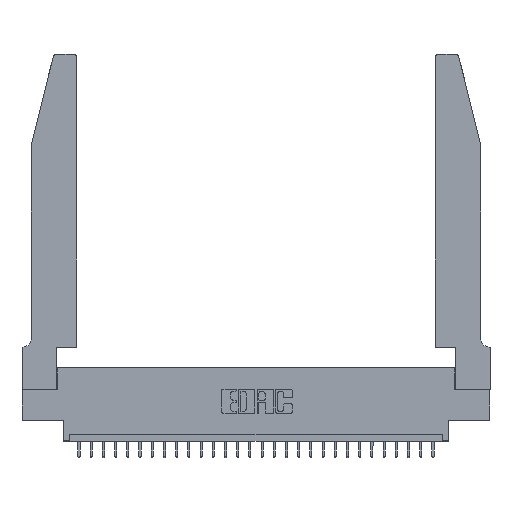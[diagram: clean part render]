
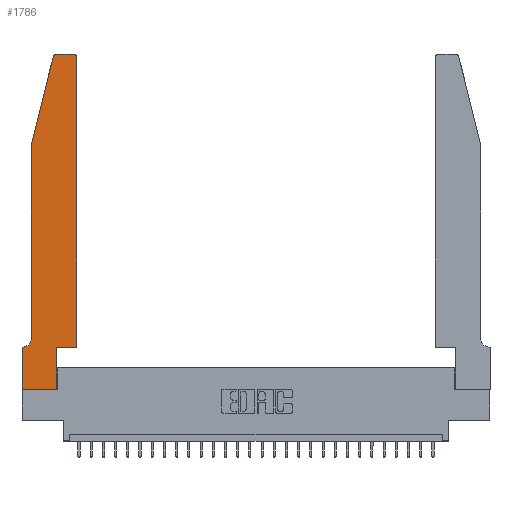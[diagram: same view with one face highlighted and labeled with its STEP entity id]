
A CAD part, top view. The second image highlights one B-rep face of the part: STEP entity #1786.
In plain terms, the highlighted planar face has unit normal (0, 0, 1).
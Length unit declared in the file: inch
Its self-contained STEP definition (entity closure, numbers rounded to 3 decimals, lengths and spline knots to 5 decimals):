
#113 = VERTEX_POINT ( 'NONE', #26144 ) ;
#346 = ORIENTED_EDGE ( 'NONE', *, *, #4771, .T. ) ;
#759 = LINE ( 'NONE', #21022, #28540 ) ;
#939 = CARTESIAN_POINT ( 'NONE',  ( 0., 0., 0.37 ) ) ;
#1081 = VECTOR ( 'NONE', #6159, 39.37008 ) ;
#1107 = EDGE_CURVE ( 'NONE', #24085, #16283, #13024, .T. ) ;
#1116 = EDGE_CURVE ( 'NONE', #14384, #13905, #27344, .T. ) ;
#1422 = CARTESIAN_POINT ( 'NONE',  ( 0.0755, 2., 0.37 ) ) ;
#1423 = LINE ( 'NONE', #18894, #9993 ) ;
#1582 = CARTESIAN_POINT ( 'NONE',  ( 0.0755, 2., 0.37 ) ) ;
#1786 = ADVANCED_FACE ( 'NONE', ( #25064 ), #11486, .T. ) ;
#2566 = CARTESIAN_POINT ( 'NONE',  ( 0.0055, 0.42, 0.37 ) ) ;
#2637 = EDGE_CURVE ( 'NONE', #11356, #17026, #1423, .T. ) ;
#3624 = DIRECTION ( 'NONE',  ( 0., 1., 0. ) ) ;
#3941 = CARTESIAN_POINT ( 'NONE',  ( 0.0055, 0.35, 0.37 ) ) ;
#4277 = DIRECTION ( 'NONE',  ( 0., -1., 0. ) ) ;
#4666 = VECTOR ( 'NONE', #4277, 39.37008 ) ;
#4771 = EDGE_CURVE ( 'NONE', #113, #11356, #10978, .T. ) ;
#5021 = CARTESIAN_POINT ( 'NONE',  ( 0.2865, 0.35, 0.37 ) ) ;
#5240 = VERTEX_POINT ( 'NONE', #14966 ) ;
#5389 = ORIENTED_EDGE ( 'NONE', *, *, #12467, .T. ) ;
#5430 = LINE ( 'NONE', #18927, #10160 ) ;
#5456 = DIRECTION ( 'NONE',  ( 0., 1., 0. ) ) ;
#5541 = CIRCLE ( 'NONE', #9285, 0.03 ) ;
#5639 = CARTESIAN_POINT ( 'NONE',  ( 0.284, 2.75, 0.37 ) ) ;
#6159 = DIRECTION ( 'NONE',  ( 0., -1., 0. ) ) ;
#6169 = ORIENTED_EDGE ( 'NONE', *, *, #23063, .T. ) ;
#6277 = ORIENTED_EDGE ( 'NONE', *, *, #1107, .T. ) ;
#6427 = VECTOR ( 'NONE', #3624, 39.37008 ) ;
#6808 = DIRECTION ( 'NONE',  ( 1., 0., 0. ) ) ;
#7432 = ORIENTED_EDGE ( 'NONE', *, *, #21163, .T. ) ;
#7960 = EDGE_CURVE ( 'NONE', #27214, #5240, #5430, .T. ) ;
#8190 = DIRECTION ( 'NONE',  ( 1., 0., 0. ) ) ;
#8300 = EDGE_CURVE ( 'NONE', #28111, #24085, #5541, .T. ) ;
#8770 = DIRECTION ( 'NONE',  ( -0.239, -0.971, 0. ) ) ;
#9285 = AXIS2_PLACEMENT_3D ( 'NONE', #19889, #18239, #6808 ) ;
#9444 = AXIS2_PLACEMENT_3D ( 'NONE', #2566, #28035, #25078 ) ;
#9508 = CARTESIAN_POINT ( 'NONE',  ( 0.4205, 2.75, 0.37 ) ) ;
#9993 = VECTOR ( 'NONE', #27955, 39.37008 ) ;
#10160 = VECTOR ( 'NONE', #8190, 39.37008 ) ;
#10300 = ORIENTED_EDGE ( 'NONE', *, *, #7960, .T. ) ;
#10596 = EDGE_CURVE ( 'NONE', #10987, #25394, #17300, .T. ) ;
#10978 = LINE ( 'NONE', #21729, #1081 ) ;
#10987 = VERTEX_POINT ( 'NONE', #25023 ) ;
#11010 = EDGE_CURVE ( 'NONE', #16283, #14384, #15411, .T. ) ;
#11028 = CARTESIAN_POINT ( 'NONE',  ( 0.25487, 2.72718, 0.37 ) ) ;
#11356 = VERTEX_POINT ( 'NONE', #939 ) ;
#11486 = PLANE ( 'NONE',  #28354 ) ;
#12087 = DIRECTION ( 'NONE',  ( -1., 0., 0. ) ) ;
#12219 = ORIENTED_EDGE ( 'NONE', *, *, #10596, .T. ) ;
#12467 = EDGE_CURVE ( 'NONE', #5240, #10987, #15061, .T. ) ;
#13024 = LINE ( 'NONE', #1582, #20252 ) ;
#13569 = AXIS2_PLACEMENT_3D ( 'NONE', #17232, #15301, #26095 ) ;
#13905 = VERTEX_POINT ( 'NONE', #3941 ) ;
#14140 = CARTESIAN_POINT ( 'NONE',  ( 0., 0.35, 0.37 ) ) ;
#14181 = LINE ( 'NONE', #18862, #22955 ) ;
#14384 = VERTEX_POINT ( 'NONE', #16089 ) ;
#14966 = CARTESIAN_POINT ( 'NONE',  ( 0.4505, 0.35, 0.37 ) ) ;
#15061 = LINE ( 'NONE', #28258, #6427 ) ;
#15301 = DIRECTION ( 'NONE',  ( 0., 0., 1. ) ) ;
#15411 = LINE ( 'NONE', #24442, #4666 ) ;
#16089 = CARTESIAN_POINT ( 'NONE',  ( 0.0755, 0.42, 0.37 ) ) ;
#16283 = VERTEX_POINT ( 'NONE', #1422 ) ;
#16498 = DIRECTION ( 'NONE',  ( 1., 0., 0. ) ) ;
#17026 = VERTEX_POINT ( 'NONE', #25400 ) ;
#17232 = CARTESIAN_POINT ( 'NONE',  ( 0.4205, 2.72, 0.37 ) ) ;
#17300 = CIRCLE ( 'NONE', #13569, 0.03 ) ;
#18239 = DIRECTION ( 'NONE',  ( 0., 0., 1. ) ) ;
#18862 = CARTESIAN_POINT ( 'NONE',  ( 0.2605, 2.75, 0.37 ) ) ;
#18894 = CARTESIAN_POINT ( 'NONE',  ( 0., 0., 0.37 ) ) ;
#18927 = CARTESIAN_POINT ( 'NONE',  ( 0.4505, 0.35, 0.37 ) ) ;
#18991 = CARTESIAN_POINT ( 'NONE',  ( 0.0755, 0.35, 0.37 ) ) ;
#19889 = CARTESIAN_POINT ( 'NONE',  ( 0.284, 2.72, 0.37 ) ) ;
#20252 = VECTOR ( 'NONE', #8770, 39.37008 ) ;
#20440 = ORIENTED_EDGE ( 'NONE', *, *, #1116, .T. ) ;
#21022 = CARTESIAN_POINT ( 'NONE',  ( 0.2865, 0.35, 0.37 ) ) ;
#21163 = EDGE_CURVE ( 'NONE', #25394, #28111, #14181, .T. ) ;
#21257 = ORIENTED_EDGE ( 'NONE', *, *, #11010, .T. ) ;
#21729 = CARTESIAN_POINT ( 'NONE',  ( 0., 0., 0.37 ) ) ;
#22814 = VECTOR ( 'NONE', #12087, 39.37008 ) ;
#22955 = VECTOR ( 'NONE', #25975, 39.37008 ) ;
#23063 = EDGE_CURVE ( 'NONE', #13905, #113, #23875, .T. ) ;
#23726 = EDGE_CURVE ( 'NONE', #17026, #27214, #759, .T. ) ;
#23875 = LINE ( 'NONE', #18991, #22814 ) ;
#24085 = VERTEX_POINT ( 'NONE', #11028 ) ;
#24242 = EDGE_LOOP ( 'NONE', ( #7432, #28319, #6277, #21257, #20440, #6169, #346, #29160, #25777, #10300, #5389, #12219 ) ) ;
#24442 = CARTESIAN_POINT ( 'NONE',  ( 0.0755, 2., 0.37 ) ) ;
#25023 = CARTESIAN_POINT ( 'NONE',  ( 0.4505, 2.72, 0.37 ) ) ;
#25064 = FACE_OUTER_BOUND ( 'NONE', #24242, .T. ) ;
#25078 = DIRECTION ( 'NONE',  ( -1., 0., 0. ) ) ;
#25341 = DIRECTION ( 'NONE',  ( 0., 0., 1. ) ) ;
#25394 = VERTEX_POINT ( 'NONE', #9508 ) ;
#25400 = CARTESIAN_POINT ( 'NONE',  ( 0.2865, 0., 0.37 ) ) ;
#25777 = ORIENTED_EDGE ( 'NONE', *, *, #23726, .T. ) ;
#25975 = DIRECTION ( 'NONE',  ( -1., 0., 0. ) ) ;
#26095 = DIRECTION ( 'NONE',  ( 1., 0., 0. ) ) ;
#26144 = CARTESIAN_POINT ( 'NONE',  ( 0., 0.35, 0.37 ) ) ;
#27214 = VERTEX_POINT ( 'NONE', #5021 ) ;
#27344 = CIRCLE ( 'NONE', #9444, 0.07 ) ;
#27955 = DIRECTION ( 'NONE',  ( 1., 0., 0. ) ) ;
#28035 = DIRECTION ( 'NONE',  ( 0., 0., -1. ) ) ;
#28111 = VERTEX_POINT ( 'NONE', #5639 ) ;
#28258 = CARTESIAN_POINT ( 'NONE',  ( 0.4505, 0.35, 0.37 ) ) ;
#28319 = ORIENTED_EDGE ( 'NONE', *, *, #8300, .T. ) ;
#28354 = AXIS2_PLACEMENT_3D ( 'NONE', #14140, #25341, #16498 ) ;
#28540 = VECTOR ( 'NONE', #5456, 39.37008 ) ;
#29160 = ORIENTED_EDGE ( 'NONE', *, *, #2637, .T. ) ;
